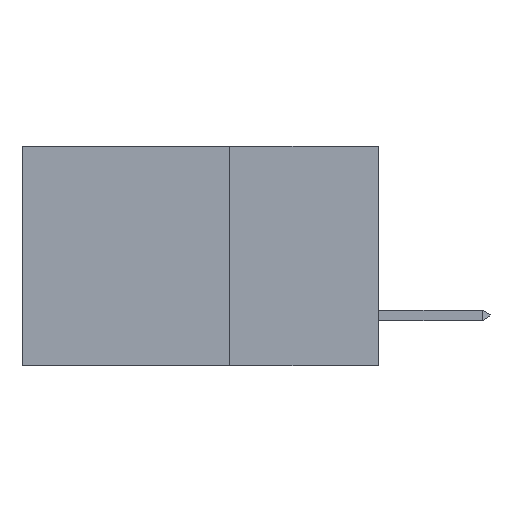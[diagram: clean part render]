
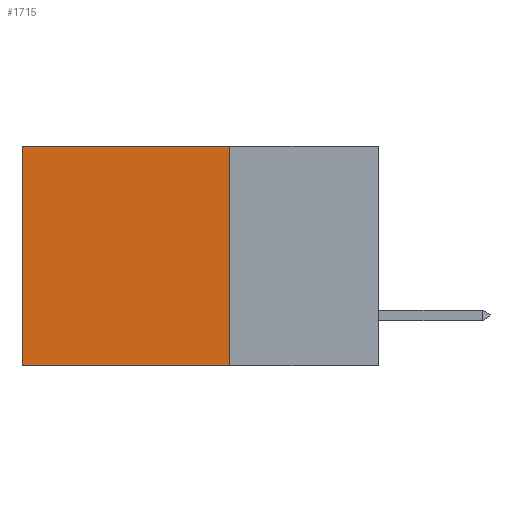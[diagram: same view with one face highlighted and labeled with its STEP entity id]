
A CAD part, left-side view. The second image highlights one B-rep face of the part: STEP entity #1715.
In plain terms, the highlighted planar face has unit normal (-1, 0, 0).
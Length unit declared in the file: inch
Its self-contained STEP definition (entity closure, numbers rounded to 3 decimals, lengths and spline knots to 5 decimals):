
#1066 = EDGE_CURVE ( 'NONE', #9009, #1283, #25770, .T. ) ;
#1283 = VERTEX_POINT ( 'NONE', #11531 ) ;
#1685 = VECTOR ( 'NONE', #9840, 39.37008 ) ;
#1715 = ADVANCED_FACE ( 'NONE', ( #14555 ), #16954, .F. ) ;
#2149 = VECTOR ( 'NONE', #18673, 39.37008 ) ;
#2762 = EDGE_CURVE ( 'NONE', #11058, #1283, #26904, .T. ) ;
#4443 = EDGE_CURVE ( 'NONE', #23239, #11058, #11324, .T. ) ;
#6247 = DIRECTION ( 'NONE',  ( 0., 0., -1. ) ) ;
#7531 = ORIENTED_EDGE ( 'NONE', *, *, #4443, .F. ) ;
#8619 = CARTESIAN_POINT ( 'NONE',  ( 0.298, 0.25, 0. ) ) ;
#9009 = VERTEX_POINT ( 'NONE', #29024 ) ;
#9840 = DIRECTION ( 'NONE',  ( 0., 0., -1. ) ) ;
#10415 = VECTOR ( 'NONE', #22527, 39.37008 ) ;
#10619 = EDGE_CURVE ( 'NONE', #23239, #9009, #11125, .T. ) ;
#11058 = VERTEX_POINT ( 'NONE', #14829 ) ;
#11125 = LINE ( 'NONE', #29266, #10415 ) ;
#11324 = LINE ( 'NONE', #8619, #22883 ) ;
#11531 = CARTESIAN_POINT ( 'NONE',  ( 0.298, 0.6, -0.37 ) ) ;
#14555 = FACE_OUTER_BOUND ( 'NONE', #29441, .T. ) ;
#14829 = CARTESIAN_POINT ( 'NONE',  ( 0.298, 0.25, -0.37 ) ) ;
#15326 = ORIENTED_EDGE ( 'NONE', *, *, #2762, .F. ) ;
#16954 = PLANE ( 'NONE',  #26999 ) ;
#18643 = CARTESIAN_POINT ( 'NONE',  ( 0.298, 0.25, -0.37 ) ) ;
#18673 = DIRECTION ( 'NONE',  ( 0., 1., 0. ) ) ;
#20416 = ORIENTED_EDGE ( 'NONE', *, *, #1066, .T. ) ;
#22044 = ORIENTED_EDGE ( 'NONE', *, *, #10619, .T. ) ;
#22527 = DIRECTION ( 'NONE',  ( 0., 1., 0. ) ) ;
#22883 = VECTOR ( 'NONE', #6247, 39.37008 ) ;
#23239 = VERTEX_POINT ( 'NONE', #29307 ) ;
#23949 = CARTESIAN_POINT ( 'NONE',  ( 0.298, 0.25, 0. ) ) ;
#24436 = DIRECTION ( 'NONE',  ( 0., 0., -1. ) ) ;
#24867 = DIRECTION ( 'NONE',  ( 1., 0., 0. ) ) ;
#25770 = LINE ( 'NONE', #26146, #1685 ) ;
#26146 = CARTESIAN_POINT ( 'NONE',  ( 0.298, 0.6, 0. ) ) ;
#26904 = LINE ( 'NONE', #18643, #2149 ) ;
#26999 = AXIS2_PLACEMENT_3D ( 'NONE', #23949, #24867, #24436 ) ;
#29024 = CARTESIAN_POINT ( 'NONE',  ( 0.298, 0.6, 0. ) ) ;
#29266 = CARTESIAN_POINT ( 'NONE',  ( 0.298, 0.25, 0. ) ) ;
#29307 = CARTESIAN_POINT ( 'NONE',  ( 0.298, 0.25, 0. ) ) ;
#29441 = EDGE_LOOP ( 'NONE', ( #20416, #15326, #7531, #22044 ) ) ;
